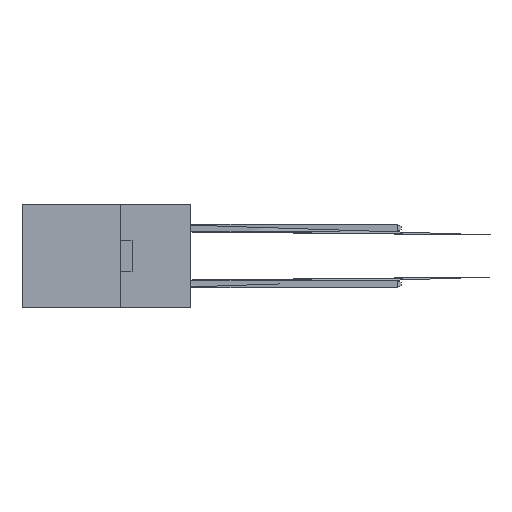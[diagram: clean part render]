
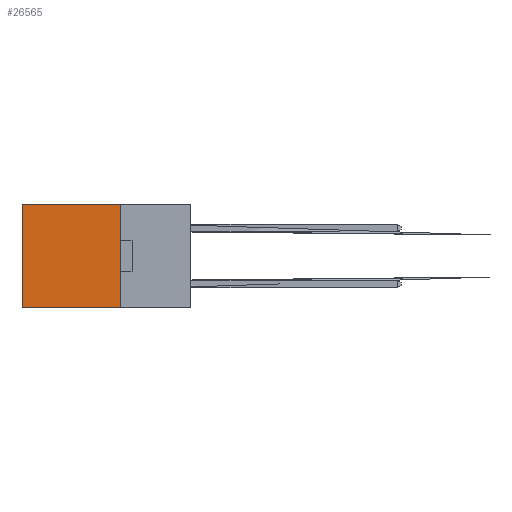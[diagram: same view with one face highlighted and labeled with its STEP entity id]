
A CAD part, left-side view. The second image highlights one B-rep face of the part: STEP entity #26565.
In plain terms, the highlighted planar face has unit normal (-1, 0, 0).
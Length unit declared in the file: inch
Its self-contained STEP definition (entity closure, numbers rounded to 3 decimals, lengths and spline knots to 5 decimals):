
#540 = CARTESIAN_POINT ( 'NONE',  ( 0.2615, 0.25, 0. ) ) ;
#2329 = CARTESIAN_POINT ( 'NONE',  ( 0.2615, 0.25, -0.37 ) ) ;
#3753 = PLANE ( 'NONE',  #5425 ) ;
#5385 = VECTOR ( 'NONE', #25911, 39.37008 ) ;
#5425 = AXIS2_PLACEMENT_3D ( 'NONE', #21386, #20821, #5660 ) ;
#5660 = DIRECTION ( 'NONE',  ( 0., 0., -1. ) ) ;
#8955 = VECTOR ( 'NONE', #20115, 39.37008 ) ;
#9041 = VECTOR ( 'NONE', #12503, 39.37008 ) ;
#9341 = LINE ( 'NONE', #17429, #18876 ) ;
#10133 = VERTEX_POINT ( 'NONE', #13881 ) ;
#10157 = EDGE_CURVE ( 'NONE', #17987, #10133, #9341, .T. ) ;
#10861 = DIRECTION ( 'NONE',  ( 0., 1., 0. ) ) ;
#11084 = LINE ( 'NONE', #2329, #8955 ) ;
#11377 = ORIENTED_EDGE ( 'NONE', *, *, #22013, .F. ) ;
#12503 = DIRECTION ( 'NONE',  ( 0., 1., 0. ) ) ;
#13603 = CARTESIAN_POINT ( 'NONE',  ( 0.2615, 0.25, -0.37 ) ) ;
#13881 = CARTESIAN_POINT ( 'NONE',  ( 0.2615, 0.6, -0.37 ) ) ;
#14711 = ORIENTED_EDGE ( 'NONE', *, *, #25571, .T. ) ;
#17335 = VERTEX_POINT ( 'NONE', #23967 ) ;
#17429 = CARTESIAN_POINT ( 'NONE',  ( 0.2615, 0.25, -0.37 ) ) ;
#17987 = VERTEX_POINT ( 'NONE', #13603 ) ;
#18486 = LINE ( 'NONE', #28484, #9041 ) ;
#18876 = VECTOR ( 'NONE', #10861, 39.37008 ) ;
#20115 = DIRECTION ( 'NONE',  ( 0., 0., -1. ) ) ;
#20821 = DIRECTION ( 'NONE',  ( 1., 0., 0. ) ) ;
#20849 = ORIENTED_EDGE ( 'NONE', *, *, #10157, .F. ) ;
#21386 = CARTESIAN_POINT ( 'NONE',  ( 0.2615, 0.25, -0.37 ) ) ;
#22013 = EDGE_CURVE ( 'NONE', #27858, #17987, #11084, .T. ) ;
#23584 = CARTESIAN_POINT ( 'NONE',  ( 0.2615, 0.6, -0.37 ) ) ;
#23967 = CARTESIAN_POINT ( 'NONE',  ( 0.2615, 0.6, 0. ) ) ;
#24138 = EDGE_CURVE ( 'NONE', #27858, #17335, #18486, .T. ) ;
#25571 = EDGE_CURVE ( 'NONE', #17335, #10133, #27661, .T. ) ;
#25911 = DIRECTION ( 'NONE',  ( 0., 0., -1. ) ) ;
#26042 = ORIENTED_EDGE ( 'NONE', *, *, #24138, .T. ) ;
#26565 = ADVANCED_FACE ( 'NONE', ( #27486 ), #3753, .F. ) ;
#27486 = FACE_OUTER_BOUND ( 'NONE', #27994, .T. ) ;
#27661 = LINE ( 'NONE', #23584, #5385 ) ;
#27858 = VERTEX_POINT ( 'NONE', #540 ) ;
#27994 = EDGE_LOOP ( 'NONE', ( #14711, #20849, #11377, #26042 ) ) ;
#28484 = CARTESIAN_POINT ( 'NONE',  ( 0.2615, 0.25, 0. ) ) ;
